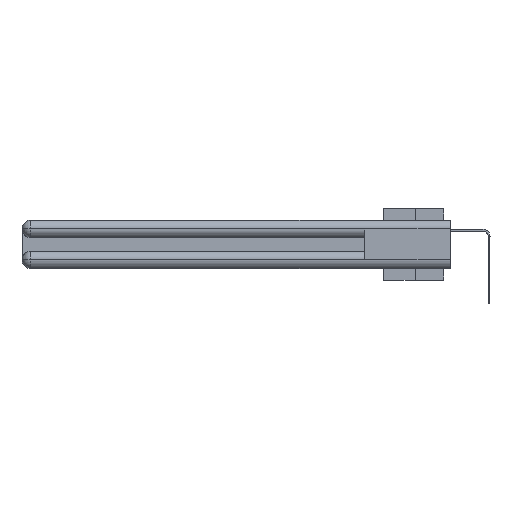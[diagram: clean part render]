
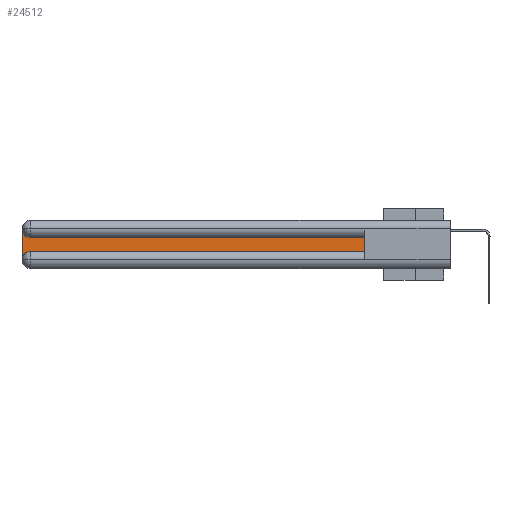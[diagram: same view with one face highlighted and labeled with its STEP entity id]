
A CAD part, left-side view. The second image highlights one B-rep face of the part: STEP entity #24512.
In plain terms, the highlighted planar face has unit normal (-1, 0, 0).
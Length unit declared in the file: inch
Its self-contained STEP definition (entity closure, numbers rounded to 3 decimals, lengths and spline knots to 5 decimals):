
#467 = CARTESIAN_POINT ( 'NONE',  ( 0.075, 0.6, -0.2175 ) ) ;
#1937 = ORIENTED_EDGE ( 'NONE', *, *, #30571, .T. ) ;
#2655 = CARTESIAN_POINT ( 'NONE',  ( 0.075, 0.6, -0.2175 ) ) ;
#2755 = CARTESIAN_POINT ( 'NONE',  ( 0.075, 0.6, -0.1225 ) ) ;
#3265 = AXIS2_PLACEMENT_3D ( 'NONE', #3761, #3878, #15522 ) ;
#3314 = DIRECTION ( 'NONE',  ( 1., 0., 0. ) ) ;
#3761 = CARTESIAN_POINT ( 'NONE',  ( 0.075, 3., -0.1225 ) ) ;
#3878 = DIRECTION ( 'NONE',  ( 1., 0., 0. ) ) ;
#6340 = CARTESIAN_POINT ( 'NONE',  ( 0.075, 3., -0.0625 ) ) ;
#7277 = VERTEX_POINT ( 'NONE', #31096 ) ;
#7956 = VECTOR ( 'NONE', #24645, 39.37008 ) ;
#8447 = EDGE_CURVE ( 'NONE', #7277, #9847, #30037, .T. ) ;
#9847 = VERTEX_POINT ( 'NONE', #6340 ) ;
#11956 = VERTEX_POINT ( 'NONE', #2755 ) ;
#12207 = DIRECTION ( 'NONE',  ( 1., 0., 0. ) ) ;
#13722 = EDGE_CURVE ( 'NONE', #14640, #11956, #29452, .T. ) ;
#14640 = VERTEX_POINT ( 'NONE', #16070 ) ;
#15115 = VERTEX_POINT ( 'NONE', #26523 ) ;
#15522 = DIRECTION ( 'NONE',  ( 0., 0., -1. ) ) ;
#15532 = EDGE_CURVE ( 'NONE', #15115, #14640, #27609, .T. ) ;
#16070 = CARTESIAN_POINT ( 'NONE',  ( 0.075, 0.6, -0.2175 ) ) ;
#17355 = EDGE_CURVE ( 'NONE', #9847, #27698, #17384, .T. ) ;
#17384 = LINE ( 'NONE', #21185, #37984 ) ;
#17551 = ORIENTED_EDGE ( 'NONE', *, *, #25772, .T. ) ;
#17677 = DIRECTION ( 'NONE',  ( 0., -1., 0. ) ) ;
#17882 = LINE ( 'NONE', #22181, #34235 ) ;
#18145 = CIRCLE ( 'NONE', #24995, 0.06 ) ;
#18225 = ORIENTED_EDGE ( 'NONE', *, *, #15532, .T. ) ;
#20517 = DIRECTION ( 'NONE',  ( 0., 0., -1. ) ) ;
#21185 = CARTESIAN_POINT ( 'NONE',  ( 0.075, 3., -0.2175 ) ) ;
#21247 = CARTESIAN_POINT ( 'NONE',  ( 0.075, 2.94, -0.0625 ) ) ;
#22181 = CARTESIAN_POINT ( 'NONE',  ( 0.075, 0.6, -0.1225 ) ) ;
#22581 = CARTESIAN_POINT ( 'NONE',  ( 0.075, 3., -0.2775 ) ) ;
#23774 = ORIENTED_EDGE ( 'NONE', *, *, #8447, .T. ) ;
#24512 = ADVANCED_FACE ( 'NONE', ( #24533 ), #27693, .F. ) ;
#24533 = FACE_OUTER_BOUND ( 'NONE', #24654, .T. ) ;
#24645 = DIRECTION ( 'NONE',  ( 0., 0., 1. ) ) ;
#24654 = EDGE_LOOP ( 'NONE', ( #17551, #23774, #37837, #1937, #18225, #33995 ) ) ;
#24995 = AXIS2_PLACEMENT_3D ( 'NONE', #32808, #12207, #20517 ) ;
#25772 = EDGE_CURVE ( 'NONE', #11956, #7277, #17882, .T. ) ;
#26523 = CARTESIAN_POINT ( 'NONE',  ( 0.075, 2.94, -0.2175 ) ) ;
#27197 = DIRECTION ( 'NONE',  ( 0., 0., -1. ) ) ;
#27609 = LINE ( 'NONE', #2655, #37884 ) ;
#27665 = DIRECTION ( 'NONE',  ( 0., 1., 0. ) ) ;
#27693 = PLANE ( 'NONE',  #3265 ) ;
#27698 = VERTEX_POINT ( 'NONE', #22581 ) ;
#29452 = LINE ( 'NONE', #467, #7956 ) ;
#30037 = CIRCLE ( 'NONE', #35025, 0.06 ) ;
#30571 = EDGE_CURVE ( 'NONE', #27698, #15115, #18145, .T. ) ;
#31096 = CARTESIAN_POINT ( 'NONE',  ( 0.075, 2.94, -0.1225 ) ) ;
#32808 = CARTESIAN_POINT ( 'NONE',  ( 0.075, 2.94, -0.2775 ) ) ;
#33995 = ORIENTED_EDGE ( 'NONE', *, *, #13722, .T. ) ;
#34235 = VECTOR ( 'NONE', #27665, 39.37008 ) ;
#35025 = AXIS2_PLACEMENT_3D ( 'NONE', #21247, #3314, #38762 ) ;
#37837 = ORIENTED_EDGE ( 'NONE', *, *, #17355, .T. ) ;
#37884 = VECTOR ( 'NONE', #17677, 39.37008 ) ;
#37984 = VECTOR ( 'NONE', #27197, 39.37008 ) ;
#38762 = DIRECTION ( 'NONE',  ( 0., 0., -1. ) ) ;
